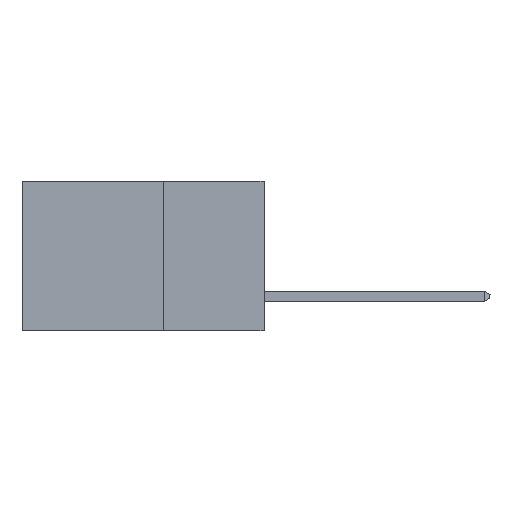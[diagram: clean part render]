
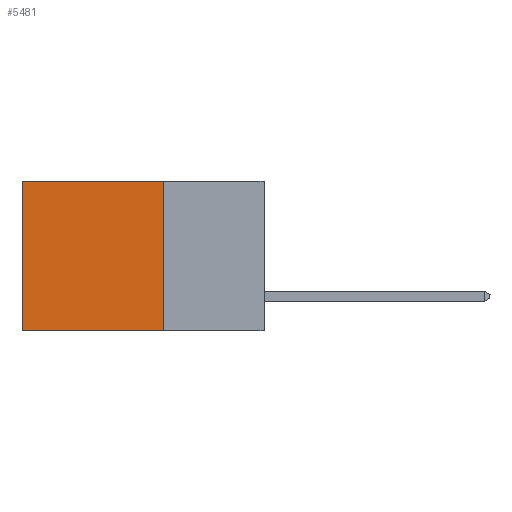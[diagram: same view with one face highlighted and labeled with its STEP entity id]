
A CAD part, left-side view. The second image highlights one B-rep face of the part: STEP entity #5481.
In plain terms, the highlighted planar face has unit normal (-1, 0, 0).
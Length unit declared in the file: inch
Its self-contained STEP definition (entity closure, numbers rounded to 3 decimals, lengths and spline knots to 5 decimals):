
#341 = DIRECTION ( 'NONE',  ( 0., 0., -1. ) ) ;
#651 = VERTEX_POINT ( 'NONE', #18645 ) ;
#799 = LINE ( 'NONE', #10849, #2272 ) ;
#2019 = LINE ( 'NONE', #18988, #9450 ) ;
#2166 = ORIENTED_EDGE ( 'NONE', *, *, #5067, .T. ) ;
#2272 = VECTOR ( 'NONE', #12184, 39.37008 ) ;
#3713 = VECTOR ( 'NONE', #8685, 39.37008 ) ;
#3967 = DIRECTION ( 'NONE',  ( 0., 0., -1. ) ) ;
#4037 = VECTOR ( 'NONE', #21427, 39.37008 ) ;
#4054 = DIRECTION ( 'NONE',  ( 1., 0., 0. ) ) ;
#4084 = LINE ( 'NONE', #5418, #3713 ) ;
#4845 = EDGE_LOOP ( 'NONE', ( #2166, #16110, #19292, #8517 ) ) ;
#4935 = EDGE_CURVE ( 'NONE', #20665, #651, #4084, .T. ) ;
#5067 = EDGE_CURVE ( 'NONE', #15383, #14646, #2019, .T. ) ;
#5418 = CARTESIAN_POINT ( 'NONE',  ( 0.2615, 0.25, -0.37 ) ) ;
#5481 = ADVANCED_FACE ( 'NONE', ( #20679 ), #5708, .F. ) ;
#5708 = PLANE ( 'NONE',  #11078 ) ;
#7905 = CARTESIAN_POINT ( 'NONE',  ( 0.2615, 0.6, 0. ) ) ;
#8517 = ORIENTED_EDGE ( 'NONE', *, *, #17473, .T. ) ;
#8685 = DIRECTION ( 'NONE',  ( 0., 0., -1. ) ) ;
#9450 = VECTOR ( 'NONE', #3967, 39.37008 ) ;
#10849 = CARTESIAN_POINT ( 'NONE',  ( 0.2615, 0.25, -0.37 ) ) ;
#11078 = AXIS2_PLACEMENT_3D ( 'NONE', #12382, #4054, #341 ) ;
#12184 = DIRECTION ( 'NONE',  ( 0., 1., 0. ) ) ;
#12382 = CARTESIAN_POINT ( 'NONE',  ( 0.2615, 0.25, -0.37 ) ) ;
#13016 = LINE ( 'NONE', #14777, #4037 ) ;
#14007 = EDGE_CURVE ( 'NONE', #651, #14646, #799, .T. ) ;
#14646 = VERTEX_POINT ( 'NONE', #19684 ) ;
#14777 = CARTESIAN_POINT ( 'NONE',  ( 0.2615, 0.25, 0. ) ) ;
#15383 = VERTEX_POINT ( 'NONE', #7905 ) ;
#16110 = ORIENTED_EDGE ( 'NONE', *, *, #14007, .F. ) ;
#17368 = CARTESIAN_POINT ( 'NONE',  ( 0.2615, 0.25, 0. ) ) ;
#17473 = EDGE_CURVE ( 'NONE', #20665, #15383, #13016, .T. ) ;
#18645 = CARTESIAN_POINT ( 'NONE',  ( 0.2615, 0.25, -0.37 ) ) ;
#18988 = CARTESIAN_POINT ( 'NONE',  ( 0.2615, 0.6, -0.37 ) ) ;
#19292 = ORIENTED_EDGE ( 'NONE', *, *, #4935, .F. ) ;
#19684 = CARTESIAN_POINT ( 'NONE',  ( 0.2615, 0.6, -0.37 ) ) ;
#20665 = VERTEX_POINT ( 'NONE', #17368 ) ;
#20679 = FACE_OUTER_BOUND ( 'NONE', #4845, .T. ) ;
#21427 = DIRECTION ( 'NONE',  ( 0., 1., 0. ) ) ;
